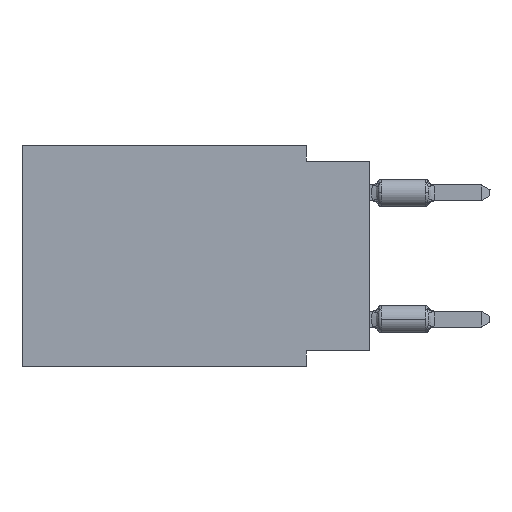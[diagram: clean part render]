
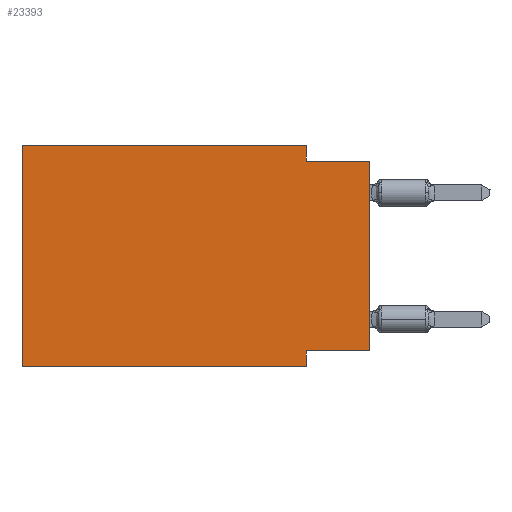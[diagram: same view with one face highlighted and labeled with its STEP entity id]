
A CAD part, left-side view. The second image highlights one B-rep face of the part: STEP entity #23393.
In plain terms, the highlighted planar face has unit normal (-1, 0, 0).
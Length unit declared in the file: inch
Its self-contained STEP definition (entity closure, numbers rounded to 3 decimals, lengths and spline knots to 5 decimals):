
#5 = ORIENTED_EDGE ( 'NONE', *, *, #22920, .F. ) ;
#150 = VERTEX_POINT ( 'NONE', #24235 ) ;
#416 = LINE ( 'NONE', #27653, #29255 ) ;
#1573 = VECTOR ( 'NONE', #11324, 39.37008 ) ;
#2170 = DIRECTION ( 'NONE',  ( 0., 0., 1. ) ) ;
#2858 = EDGE_CURVE ( 'NONE', #150, #18161, #20862, .T. ) ;
#2962 = ORIENTED_EDGE ( 'NONE', *, *, #22288, .F. ) ;
#2963 = PLANE ( 'NONE',  #26497 ) ;
#3203 = DIRECTION ( 'NONE',  ( 0., -1., 0. ) ) ;
#3865 = CARTESIAN_POINT ( 'NONE',  ( 0., 0.1, -0.35 ) ) ;
#4306 = VECTOR ( 'NONE', #23894, 39.37008 ) ;
#4393 = ORIENTED_EDGE ( 'NONE', *, *, #11032, .F. ) ;
#4481 = VECTOR ( 'NONE', #19455, 39.37008 ) ;
#4792 = DIRECTION ( 'NONE',  ( 0., 0., -1. ) ) ;
#5081 = CARTESIAN_POINT ( 'NONE',  ( 0., 0.1, -0.025 ) ) ;
#5355 = ORIENTED_EDGE ( 'NONE', *, *, #5933, .F. ) ;
#5933 = EDGE_CURVE ( 'NONE', #9608, #8918, #416, .T. ) ;
#8918 = VERTEX_POINT ( 'NONE', #5081 ) ;
#9482 = LINE ( 'NONE', #31980, #24927 ) ;
#9568 = CARTESIAN_POINT ( 'NONE',  ( 0., 0., 0. ) ) ;
#9608 = VERTEX_POINT ( 'NONE', #23937 ) ;
#10455 = CARTESIAN_POINT ( 'NONE',  ( 0., 0., -0.025 ) ) ;
#10595 = DIRECTION ( 'NONE',  ( 0., 1., 0. ) ) ;
#11032 = EDGE_CURVE ( 'NONE', #20819, #9608, #9482, .T. ) ;
#11324 = DIRECTION ( 'NONE',  ( 0., 0., -1. ) ) ;
#11598 = EDGE_CURVE ( 'NONE', #29341, #27703, #17893, .T. ) ;
#11798 = LINE ( 'NONE', #3865, #1573 ) ;
#12570 = DIRECTION ( 'NONE',  ( 0., -1., 0. ) ) ;
#12653 = EDGE_CURVE ( 'NONE', #8918, #24346, #16448, .T. ) ;
#14510 = CARTESIAN_POINT ( 'NONE',  ( 0., 0.55, 0. ) ) ;
#14571 = VECTOR ( 'NONE', #2170, 39.37008 ) ;
#15026 = CARTESIAN_POINT ( 'NONE',  ( 0., 0.55, 0. ) ) ;
#15046 = ORIENTED_EDGE ( 'NONE', *, *, #11598, .F. ) ;
#15539 = CARTESIAN_POINT ( 'NONE',  ( 0., 0.55, -0.35 ) ) ;
#16324 = ORIENTED_EDGE ( 'NONE', *, *, #29365, .T. ) ;
#16448 = LINE ( 'NONE', #26323, #4306 ) ;
#16867 = LINE ( 'NONE', #9568, #4481 ) ;
#16940 = LINE ( 'NONE', #14510, #14571 ) ;
#17190 = VECTOR ( 'NONE', #10595, 39.37008 ) ;
#17892 = ORIENTED_EDGE ( 'NONE', *, *, #12653, .F. ) ;
#17893 = LINE ( 'NONE', #25185, #17190 ) ;
#17977 = CARTESIAN_POINT ( 'NONE',  ( 0., 0.1, -0.35 ) ) ;
#18161 = VERTEX_POINT ( 'NONE', #17977 ) ;
#19455 = DIRECTION ( 'NONE',  ( 0., 0., 1. ) ) ;
#19492 = ORIENTED_EDGE ( 'NONE', *, *, #2858, .T. ) ;
#20139 = FACE_OUTER_BOUND ( 'NONE', #27060, .T. ) ;
#20819 = VERTEX_POINT ( 'NONE', #15026 ) ;
#20862 = LINE ( 'NONE', #15539, #29639 ) ;
#22288 = EDGE_CURVE ( 'NONE', #27703, #18161, #11798, .T. ) ;
#22920 = EDGE_CURVE ( 'NONE', #150, #20819, #16940, .T. ) ;
#23393 = ADVANCED_FACE ( 'NONE', ( #20139 ), #2963, .F. ) ;
#23894 = DIRECTION ( 'NONE',  ( 0., -1., 0. ) ) ;
#23937 = CARTESIAN_POINT ( 'NONE',  ( 0., 0.1, 0. ) ) ;
#24235 = CARTESIAN_POINT ( 'NONE',  ( 0., 0.55, -0.35 ) ) ;
#24346 = VERTEX_POINT ( 'NONE', #10455 ) ;
#24927 = VECTOR ( 'NONE', #12570, 39.37008 ) ;
#25185 = CARTESIAN_POINT ( 'NONE',  ( 0., 0., -0.325 ) ) ;
#26323 = CARTESIAN_POINT ( 'NONE',  ( 0., 0., -0.025 ) ) ;
#26497 = AXIS2_PLACEMENT_3D ( 'NONE', #30153, #30479, #29987 ) ;
#27060 = EDGE_LOOP ( 'NONE', ( #16324, #17892, #5355, #4393, #5, #19492, #2962, #15046 ) ) ;
#27374 = CARTESIAN_POINT ( 'NONE',  ( 0., 0.1, -0.325 ) ) ;
#27653 = CARTESIAN_POINT ( 'NONE',  ( 0., 0.1, 0. ) ) ;
#27703 = VERTEX_POINT ( 'NONE', #27374 ) ;
#29255 = VECTOR ( 'NONE', #4792, 39.37008 ) ;
#29341 = VERTEX_POINT ( 'NONE', #31740 ) ;
#29365 = EDGE_CURVE ( 'NONE', #29341, #24346, #16867, .T. ) ;
#29639 = VECTOR ( 'NONE', #3203, 39.37008 ) ;
#29987 = DIRECTION ( 'NONE',  ( 0., 0., -1. ) ) ;
#30153 = CARTESIAN_POINT ( 'NONE',  ( 0., 0.55, 0. ) ) ;
#30479 = DIRECTION ( 'NONE',  ( 1., 0., 0. ) ) ;
#31740 = CARTESIAN_POINT ( 'NONE',  ( 0., 0., -0.325 ) ) ;
#31980 = CARTESIAN_POINT ( 'NONE',  ( 0., 0.55, 0. ) ) ;
